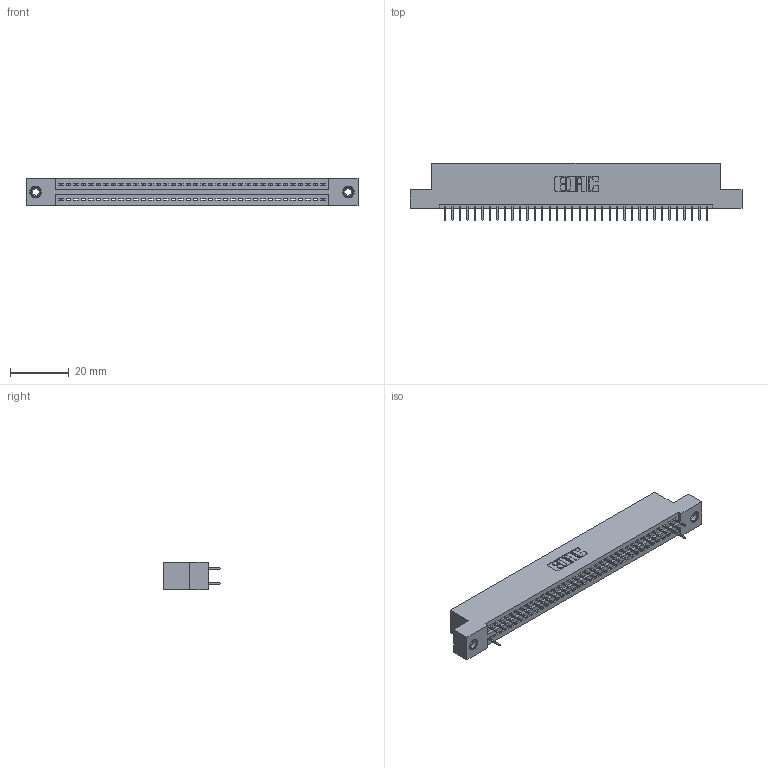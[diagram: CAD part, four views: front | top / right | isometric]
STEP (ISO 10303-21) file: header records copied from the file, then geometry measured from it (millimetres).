
FILE_DESCRIPTION (( 'STEP AP203' ), '1' );
FILE_NAME ('395-072-524-208.STEP', '2018-11-27T10:14:58', ( '' ), ( '' ), 'SwSTEP 2.0', 'SolidWorks 2016', '' );
FILE_SCHEMA (( 'CONFIG_CONTROL_DESIGN' ));
Length unit declared in the file: inch
Products named in the file (4): 345-292-001_345-293-124; 345 Part_Flush Mounting Lugs - 0.156 Dia-TI; 395-072-524-208; 345-250-001_345-250-003-102
Assembly tree (41 placements, depth 2):
  395-072-524-208
    345 Part_Flush Mounting Lugs - 0.156 Dia-TI
    345-292-001_345-293-124  x38
    345-250-001_345-250-003-102  x2
Bounding box: 112.65 x 19.35 x 9.4 mm (x, y, z)
Volume: 10516.6 mm3; surface area: 13554.9 mm2
Topology: 41 solids, 41 shells, 2510 faces, 7209 edges, 4646 vertices
Faces by surface type: plane 1832, cylinder 662, cone 12, torus 4
Entity records: 29226 total; most frequent: CARTESIAN_POINT 5033, ORIENTED_EDGE 4994, DIRECTION 4435, EDGE_CURVE 2497, LINE 2205, VECTOR 2205, VERTEX_POINT 1656, AXIS2_PLACEMENT_3D 1115
